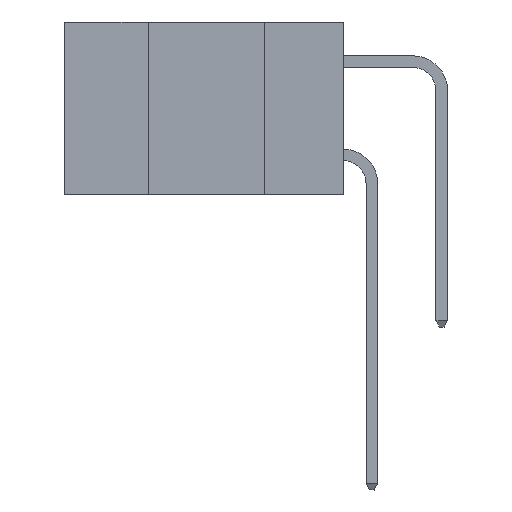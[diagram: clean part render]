
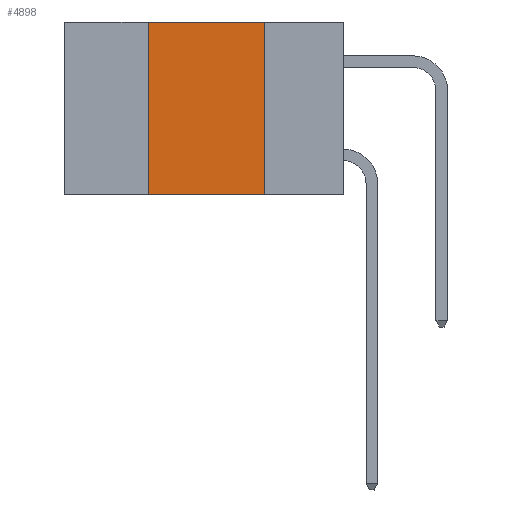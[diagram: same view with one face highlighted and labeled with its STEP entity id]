
A CAD part, left-side view. The second image highlights one B-rep face of the part: STEP entity #4898.
In plain terms, the highlighted planar face has unit normal (-1, 0, 0).
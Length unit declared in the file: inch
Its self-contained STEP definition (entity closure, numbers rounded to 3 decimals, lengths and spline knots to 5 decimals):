
#234 = VECTOR ( 'NONE', #11397, 39.37008 ) ;
#495 = LINE ( 'NONE', #5220, #1863 ) ;
#990 = LINE ( 'NONE', #5707, #234 ) ;
#1588 = DIRECTION ( 'NONE',  ( 0., -1., 0. ) ) ;
#1863 = VECTOR ( 'NONE', #1588, 39.37008 ) ;
#1946 = EDGE_CURVE ( 'NONE', #14704, #10990, #495, .T. ) ;
#2158 = DIRECTION ( 'NONE',  ( 0., 0., -1. ) ) ;
#2275 = AXIS2_PLACEMENT_3D ( 'NONE', #15038, #4481, #2158 ) ;
#2397 = CARTESIAN_POINT ( 'NONE',  ( 0., 0.17, -0.37 ) ) ;
#2964 = DIRECTION ( 'NONE',  ( 0., -1., 0. ) ) ;
#3324 = EDGE_CURVE ( 'NONE', #14704, #4805, #990, .T. ) ;
#3903 = ORIENTED_EDGE ( 'NONE', *, *, #4434, .F. ) ;
#4434 = EDGE_CURVE ( 'NONE', #4805, #14771, #6443, .T. ) ;
#4481 = DIRECTION ( 'NONE',  ( 1., 0., 0. ) ) ;
#4805 = VERTEX_POINT ( 'NONE', #11256 ) ;
#4898 = ADVANCED_FACE ( 'NONE', ( #8030 ), #10326, .F. ) ;
#5220 = CARTESIAN_POINT ( 'NONE',  ( 0., 0.6, -0.37 ) ) ;
#5707 = CARTESIAN_POINT ( 'NONE',  ( 0., 0.42, -0.37 ) ) ;
#6224 = ORIENTED_EDGE ( 'NONE', *, *, #1946, .T. ) ;
#6443 = LINE ( 'NONE', #11136, #7949 ) ;
#7050 = CARTESIAN_POINT ( 'NONE',  ( 0., 0.42, -0.37 ) ) ;
#7949 = VECTOR ( 'NONE', #2964, 39.37008 ) ;
#8030 = FACE_OUTER_BOUND ( 'NONE', #13655, .T. ) ;
#8109 = LINE ( 'NONE', #2397, #11710 ) ;
#8312 = EDGE_CURVE ( 'NONE', #14771, #10990, #8109, .T. ) ;
#10111 = CARTESIAN_POINT ( 'NONE',  ( 0., 0.17, -0.37 ) ) ;
#10326 = PLANE ( 'NONE',  #2275 ) ;
#10500 = DIRECTION ( 'NONE',  ( 0., 0., -1. ) ) ;
#10990 = VERTEX_POINT ( 'NONE', #10111 ) ;
#11136 = CARTESIAN_POINT ( 'NONE',  ( 0., 0.6, 0. ) ) ;
#11256 = CARTESIAN_POINT ( 'NONE',  ( 0., 0.42, 0. ) ) ;
#11397 = DIRECTION ( 'NONE',  ( 0., 0., 1. ) ) ;
#11515 = CARTESIAN_POINT ( 'NONE',  ( 0., 0.17, 0. ) ) ;
#11710 = VECTOR ( 'NONE', #10500, 39.37008 ) ;
#11919 = ORIENTED_EDGE ( 'NONE', *, *, #3324, .F. ) ;
#13240 = ORIENTED_EDGE ( 'NONE', *, *, #8312, .F. ) ;
#13655 = EDGE_LOOP ( 'NONE', ( #13240, #3903, #11919, #6224 ) ) ;
#14704 = VERTEX_POINT ( 'NONE', #7050 ) ;
#14771 = VERTEX_POINT ( 'NONE', #11515 ) ;
#15038 = CARTESIAN_POINT ( 'NONE',  ( 0., 0.6, 0. ) ) ;
